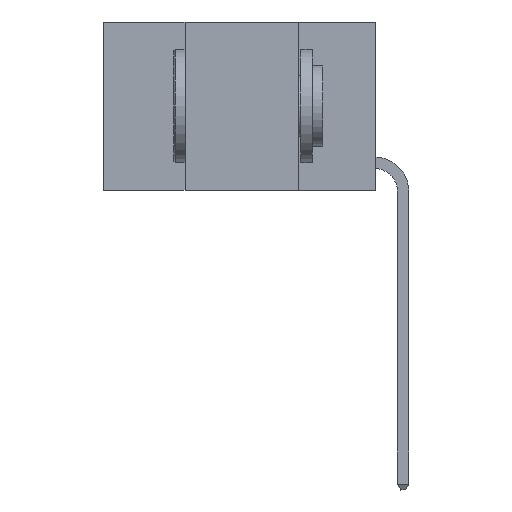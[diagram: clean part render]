
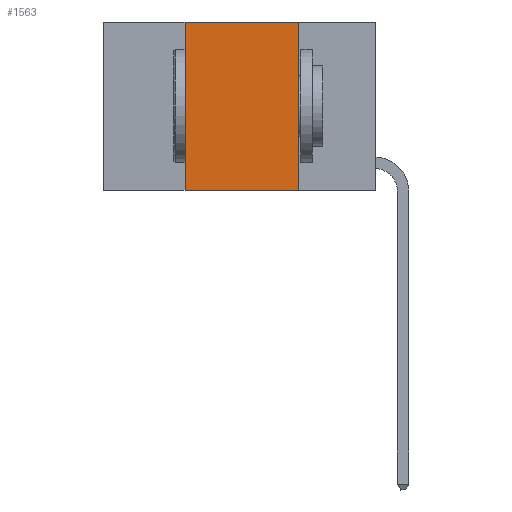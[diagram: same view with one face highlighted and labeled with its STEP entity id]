
A CAD part, left-side view. The second image highlights one B-rep face of the part: STEP entity #1563.
In plain terms, the highlighted planar face has unit normal (-1, 0, 0).
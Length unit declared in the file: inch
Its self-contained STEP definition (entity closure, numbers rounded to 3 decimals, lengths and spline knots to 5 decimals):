
#137 = EDGE_CURVE ( 'NONE', #7211, #7301, #8347, .T. ) ;
#602 = DIRECTION ( 'NONE',  ( 0., 0., 1. ) ) ;
#1094 = LINE ( 'NONE', #3833, #4072 ) ;
#1203 = DIRECTION ( 'NONE',  ( 0., -1., 0. ) ) ;
#1563 = ADVANCED_FACE ( 'NONE', ( #11194 ), #8352, .F. ) ;
#2059 = EDGE_LOOP ( 'NONE', ( #3943, #2098, #2085, #13731 ) ) ;
#2085 = ORIENTED_EDGE ( 'NONE', *, *, #13749, .F. ) ;
#2098 = ORIENTED_EDGE ( 'NONE', *, *, #10236, .F. ) ;
#2983 = CARTESIAN_POINT ( 'NONE',  ( 0., 0.17, -0.37 ) ) ;
#3701 = CARTESIAN_POINT ( 'NONE',  ( 0., 0.42, 0. ) ) ;
#3833 = CARTESIAN_POINT ( 'NONE',  ( 0., 0.6, 0. ) ) ;
#3943 = ORIENTED_EDGE ( 'NONE', *, *, #137, .F. ) ;
#4072 = VECTOR ( 'NONE', #10929, 39.37008 ) ;
#4178 = CARTESIAN_POINT ( 'NONE',  ( 0., 0.17, 0. ) ) ;
#5310 = LINE ( 'NONE', #17995, #14735 ) ;
#5466 = VECTOR ( 'NONE', #10014, 39.37008 ) ;
#6199 = LINE ( 'NONE', #3701, #14143 ) ;
#7211 = VERTEX_POINT ( 'NONE', #16665 ) ;
#7250 = CARTESIAN_POINT ( 'NONE',  ( 0., 0.6, 0. ) ) ;
#7301 = VERTEX_POINT ( 'NONE', #2983 ) ;
#7337 = DIRECTION ( 'NONE',  ( 1., 0., 0. ) ) ;
#7551 = CARTESIAN_POINT ( 'NONE',  ( 0., 0.42, -0.37 ) ) ;
#8347 = LINE ( 'NONE', #4178, #5466 ) ;
#8352 = PLANE ( 'NONE',  #16474 ) ;
#8594 = CARTESIAN_POINT ( 'NONE',  ( 0., 0.42, 0. ) ) ;
#10014 = DIRECTION ( 'NONE',  ( 0., 0., -1. ) ) ;
#10236 = EDGE_CURVE ( 'NONE', #17495, #7211, #1094, .T. ) ;
#10929 = DIRECTION ( 'NONE',  ( 0., -1., 0. ) ) ;
#11194 = FACE_OUTER_BOUND ( 'NONE', #2059, .T. ) ;
#13731 = ORIENTED_EDGE ( 'NONE', *, *, #14324, .T. ) ;
#13749 = EDGE_CURVE ( 'NONE', #14882, #17495, #6199, .T. ) ;
#13942 = DIRECTION ( 'NONE',  ( 0., 0., -1. ) ) ;
#14143 = VECTOR ( 'NONE', #602, 39.37008 ) ;
#14324 = EDGE_CURVE ( 'NONE', #14882, #7301, #5310, .T. ) ;
#14735 = VECTOR ( 'NONE', #1203, 39.37008 ) ;
#14882 = VERTEX_POINT ( 'NONE', #7551 ) ;
#16474 = AXIS2_PLACEMENT_3D ( 'NONE', #7250, #7337, #13942 ) ;
#16665 = CARTESIAN_POINT ( 'NONE',  ( 0., 0.17, 0. ) ) ;
#17495 = VERTEX_POINT ( 'NONE', #8594 ) ;
#17995 = CARTESIAN_POINT ( 'NONE',  ( 0., 0.6, -0.37 ) ) ;
